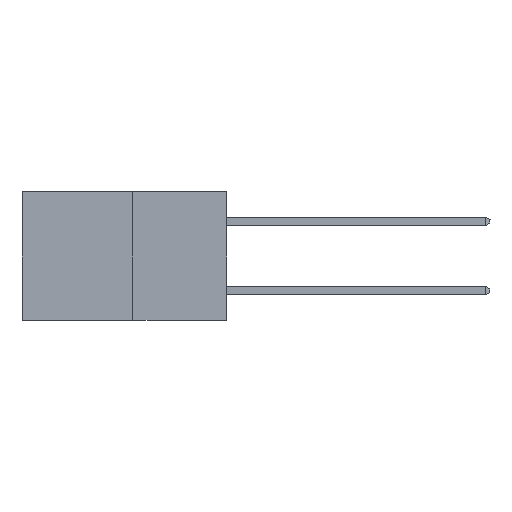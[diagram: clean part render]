
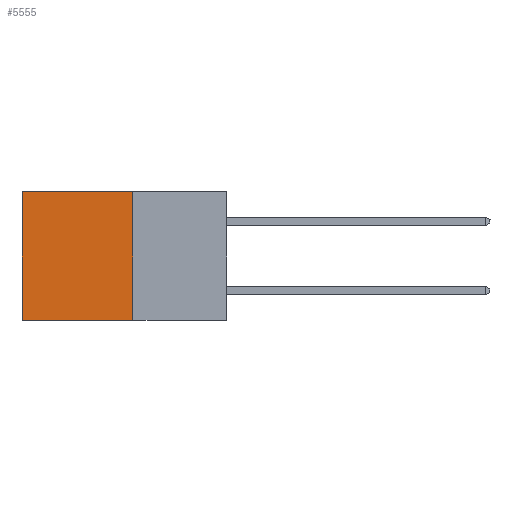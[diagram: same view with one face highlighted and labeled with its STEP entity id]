
A CAD part, left-side view. The second image highlights one B-rep face of the part: STEP entity #5555.
In plain terms, the highlighted planar face has unit normal (-1, 0, 0).
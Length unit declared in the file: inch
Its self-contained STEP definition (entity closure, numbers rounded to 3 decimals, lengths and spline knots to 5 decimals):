
#70 = LINE ( 'NONE', #3865, #22114 ) ;
#1270 = ORIENTED_EDGE ( 'NONE', *, *, #9071, .F. ) ;
#2746 = VECTOR ( 'NONE', #2754, 39.37008 ) ;
#2754 = DIRECTION ( 'NONE',  ( 0., 0., -1. ) ) ;
#3862 = ORIENTED_EDGE ( 'NONE', *, *, #19296, .F. ) ;
#3865 = CARTESIAN_POINT ( 'NONE',  ( 0.277, 0.27, -0.37 ) ) ;
#5009 = EDGE_LOOP ( 'NONE', ( #10989, #1270, #3862, #5157 ) ) ;
#5157 = ORIENTED_EDGE ( 'NONE', *, *, #25063, .T. ) ;
#5555 = ADVANCED_FACE ( 'NONE', ( #17659 ), #12447, .F. ) ;
#5904 = VECTOR ( 'NONE', #25804, 39.37008 ) ;
#5920 = VERTEX_POINT ( 'NONE', #25220 ) ;
#7090 = CARTESIAN_POINT ( 'NONE',  ( 0.277, 0.59, 0. ) ) ;
#8303 = DIRECTION ( 'NONE',  ( 0., 0., -1. ) ) ;
#8949 = LINE ( 'NONE', #22708, #10242 ) ;
#9071 = EDGE_CURVE ( 'NONE', #15948, #12762, #70, .T. ) ;
#10242 = VECTOR ( 'NONE', #8303, 39.37008 ) ;
#10989 = ORIENTED_EDGE ( 'NONE', *, *, #18392, .T. ) ;
#11565 = DIRECTION ( 'NONE',  ( 0., 0., -1. ) ) ;
#11571 = DIRECTION ( 'NONE',  ( 1., 0., 0. ) ) ;
#12092 = CARTESIAN_POINT ( 'NONE',  ( 0.277, 0.27, -0.37 ) ) ;
#12447 = PLANE ( 'NONE',  #24493 ) ;
#12762 = VERTEX_POINT ( 'NONE', #19440 ) ;
#13056 = CARTESIAN_POINT ( 'NONE',  ( 0.277, 0.27, -0.37 ) ) ;
#14277 = DIRECTION ( 'NONE',  ( 0., 1., 0. ) ) ;
#15948 = VERTEX_POINT ( 'NONE', #13056 ) ;
#17047 = LINE ( 'NONE', #23841, #5904 ) ;
#17659 = FACE_OUTER_BOUND ( 'NONE', #5009, .T. ) ;
#18392 = EDGE_CURVE ( 'NONE', #23139, #12762, #8949, .T. ) ;
#19296 = EDGE_CURVE ( 'NONE', #5920, #15948, #19298, .T. ) ;
#19298 = LINE ( 'NONE', #25241, #2746 ) ;
#19440 = CARTESIAN_POINT ( 'NONE',  ( 0.277, 0.59, -0.37 ) ) ;
#22114 = VECTOR ( 'NONE', #14277, 39.37008 ) ;
#22708 = CARTESIAN_POINT ( 'NONE',  ( 0.277, 0.59, -0.37 ) ) ;
#23139 = VERTEX_POINT ( 'NONE', #7090 ) ;
#23841 = CARTESIAN_POINT ( 'NONE',  ( 0.277, 0.27, 0. ) ) ;
#24493 = AXIS2_PLACEMENT_3D ( 'NONE', #12092, #11571, #11565 ) ;
#25063 = EDGE_CURVE ( 'NONE', #5920, #23139, #17047, .T. ) ;
#25220 = CARTESIAN_POINT ( 'NONE',  ( 0.277, 0.27, 0. ) ) ;
#25241 = CARTESIAN_POINT ( 'NONE',  ( 0.277, 0.27, -0.37 ) ) ;
#25804 = DIRECTION ( 'NONE',  ( 0., 1., 0. ) ) ;
